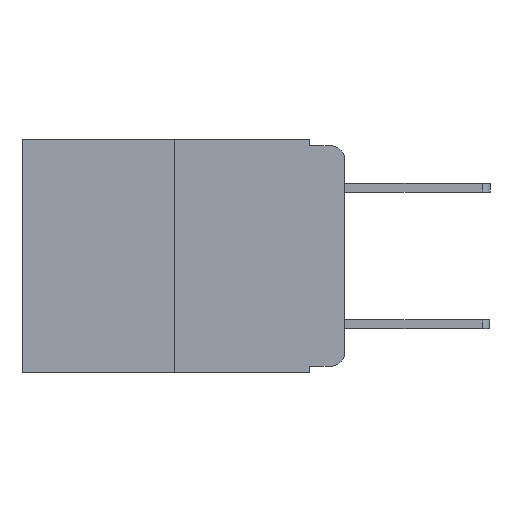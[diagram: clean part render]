
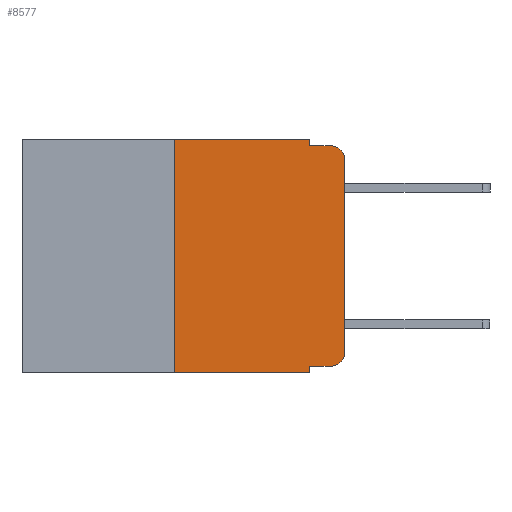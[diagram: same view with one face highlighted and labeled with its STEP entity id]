
A CAD part, left-side view. The second image highlights one B-rep face of the part: STEP entity #8577.
In plain terms, the highlighted planar face has unit normal (-1, 0, 0).
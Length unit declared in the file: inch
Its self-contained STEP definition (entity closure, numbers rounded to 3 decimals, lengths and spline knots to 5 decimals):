
#86 = EDGE_CURVE ( 'NONE', #1387, #10862, #3607, .T. ) ;
#241 = DIRECTION ( 'NONE',  ( 0., 0., -1. ) ) ;
#514 = DIRECTION ( 'NONE',  ( 0., 0., -1. ) ) ;
#557 = DIRECTION ( 'NONE',  ( 0., 0., -1. ) ) ;
#884 = CARTESIAN_POINT ( 'NONE',  ( 0., 0.051, 0. ) ) ;
#912 = VECTOR ( 'NONE', #6676, 39.37008 ) ;
#996 = ORIENTED_EDGE ( 'NONE', *, *, #6839, .F. ) ;
#1213 = LINE ( 'NONE', #5836, #912 ) ;
#1271 = VECTOR ( 'NONE', #1959, 39.37008 ) ;
#1387 = VERTEX_POINT ( 'NONE', #10732 ) ;
#1526 = DIRECTION ( 'NONE',  ( 0., -1., 0. ) ) ;
#1677 = VERTEX_POINT ( 'NONE', #6286 ) ;
#1717 = LINE ( 'NONE', #3192, #10465 ) ;
#1836 = PLANE ( 'NONE',  #3617 ) ;
#1959 = DIRECTION ( 'NONE',  ( 0., 0., 1. ) ) ;
#2155 = DIRECTION ( 'NONE',  ( 0., 0., -1. ) ) ;
#2168 = DIRECTION ( 'NONE',  ( -1., 0., 0. ) ) ;
#2172 = CARTESIAN_POINT ( 'NONE',  ( 0., 0.02, -0.03 ) ) ;
#2195 = CARTESIAN_POINT ( 'NONE',  ( 0., 0.473, 0. ) ) ;
#2405 = CARTESIAN_POINT ( 'NONE',  ( 0., 0.02, -0.333 ) ) ;
#2695 = ORIENTED_EDGE ( 'NONE', *, *, #5338, .T. ) ;
#2699 = VERTEX_POINT ( 'NONE', #2405 ) ;
#2717 = DIRECTION ( 'NONE',  ( 1., 0., 0. ) ) ;
#3094 = ORIENTED_EDGE ( 'NONE', *, *, #5093, .F. ) ;
#3158 = DIRECTION ( 'NONE',  ( -1., 0., 0. ) ) ;
#3192 = CARTESIAN_POINT ( 'NONE',  ( 0., 0.051, 0. ) ) ;
#3607 = LINE ( 'NONE', #884, #5681 ) ;
#3617 = AXIS2_PLACEMENT_3D ( 'NONE', #7880, #2717, #8708 ) ;
#4043 = ORIENTED_EDGE ( 'NONE', *, *, #8713, .F. ) ;
#4108 = CARTESIAN_POINT ( 'NONE',  ( 0., 0.25, 0. ) ) ;
#4157 = EDGE_CURVE ( 'NONE', #6738, #10862, #5843, .T. ) ;
#4356 = EDGE_CURVE ( 'NONE', #8860, #1677, #10583, .T. ) ;
#4397 = CARTESIAN_POINT ( 'NONE',  ( 0., 0., 0. ) ) ;
#4400 = CARTESIAN_POINT ( 'NONE',  ( 0., 0., -0.313 ) ) ;
#4438 = EDGE_CURVE ( 'NONE', #2699, #8860, #5134, .T. ) ;
#4764 = CARTESIAN_POINT ( 'NONE',  ( 0., 0.051, -0.343 ) ) ;
#4814 = VERTEX_POINT ( 'NONE', #4108 ) ;
#4896 = EDGE_LOOP ( 'NONE', ( #10614, #2695, #4043, #8983, #3094, #996, #6770, #7943, #9459, #10344 ) ) ;
#5035 = CARTESIAN_POINT ( 'NONE',  ( 0., 0.051, -0.01 ) ) ;
#5093 = EDGE_CURVE ( 'NONE', #4814, #6397, #6067, .T. ) ;
#5134 = CIRCLE ( 'NONE', #10412, 0.02 ) ;
#5338 = EDGE_CURVE ( 'NONE', #1677, #9386, #5941, .T. ) ;
#5553 = VERTEX_POINT ( 'NONE', #9398 ) ;
#5681 = VECTOR ( 'NONE', #557, 39.37008 ) ;
#5836 = CARTESIAN_POINT ( 'NONE',  ( 0., 0.25, 0. ) ) ;
#5840 = CARTESIAN_POINT ( 'NONE',  ( 0., 0.02, -0.313 ) ) ;
#5843 = LINE ( 'NONE', #6754, #9705 ) ;
#5941 = CIRCLE ( 'NONE', #6530, 0.02 ) ;
#6067 = LINE ( 'NONE', #2195, #10438 ) ;
#6286 = CARTESIAN_POINT ( 'NONE',  ( 0., 0., -0.03 ) ) ;
#6397 = VERTEX_POINT ( 'NONE', #11040 ) ;
#6530 = AXIS2_PLACEMENT_3D ( 'NONE', #2172, #2168, #2155 ) ;
#6539 = CARTESIAN_POINT ( 'NONE',  ( 0., 0.25, -0.343 ) ) ;
#6640 = EDGE_CURVE ( 'NONE', #1387, #2699, #7485, .T. ) ;
#6676 = DIRECTION ( 'NONE',  ( 0., 0., 1. ) ) ;
#6738 = VERTEX_POINT ( 'NONE', #6539 ) ;
#6754 = CARTESIAN_POINT ( 'NONE',  ( 0., 0.473, -0.343 ) ) ;
#6770 = ORIENTED_EDGE ( 'NONE', *, *, #4157, .T. ) ;
#6839 = EDGE_CURVE ( 'NONE', #6738, #4814, #1213, .T. ) ;
#7230 = VECTOR ( 'NONE', #8129, 39.37008 ) ;
#7307 = CARTESIAN_POINT ( 'NONE',  ( 0., 0.051, -0.333 ) ) ;
#7485 = LINE ( 'NONE', #7307, #7230 ) ;
#7732 = CARTESIAN_POINT ( 'NONE',  ( 0., 0.02, -0.01 ) ) ;
#7880 = CARTESIAN_POINT ( 'NONE',  ( 0., 0.473, 0. ) ) ;
#7943 = ORIENTED_EDGE ( 'NONE', *, *, #86, .F. ) ;
#8099 = DIRECTION ( 'NONE',  ( 0., -1., 0. ) ) ;
#8129 = DIRECTION ( 'NONE',  ( 0., -1., 0. ) ) ;
#8577 = ADVANCED_FACE ( 'NONE', ( #9272 ), #1836, .F. ) ;
#8708 = DIRECTION ( 'NONE',  ( 0., 0., -1. ) ) ;
#8713 = EDGE_CURVE ( 'NONE', #5553, #9386, #9887, .T. ) ;
#8860 = VERTEX_POINT ( 'NONE', #4400 ) ;
#8983 = ORIENTED_EDGE ( 'NONE', *, *, #10324, .F. ) ;
#9272 = FACE_OUTER_BOUND ( 'NONE', #4896, .T. ) ;
#9386 = VERTEX_POINT ( 'NONE', #7732 ) ;
#9398 = CARTESIAN_POINT ( 'NONE',  ( 0., 0.051, -0.01 ) ) ;
#9459 = ORIENTED_EDGE ( 'NONE', *, *, #6640, .T. ) ;
#9705 = VECTOR ( 'NONE', #11120, 39.37008 ) ;
#9887 = LINE ( 'NONE', #5035, #10129 ) ;
#10129 = VECTOR ( 'NONE', #1526, 39.37008 ) ;
#10324 = EDGE_CURVE ( 'NONE', #6397, #5553, #1717, .T. ) ;
#10344 = ORIENTED_EDGE ( 'NONE', *, *, #4438, .T. ) ;
#10412 = AXIS2_PLACEMENT_3D ( 'NONE', #5840, #3158, #241 ) ;
#10438 = VECTOR ( 'NONE', #8099, 39.37008 ) ;
#10465 = VECTOR ( 'NONE', #514, 39.37008 ) ;
#10583 = LINE ( 'NONE', #4397, #1271 ) ;
#10614 = ORIENTED_EDGE ( 'NONE', *, *, #4356, .T. ) ;
#10732 = CARTESIAN_POINT ( 'NONE',  ( 0., 0.051, -0.333 ) ) ;
#10862 = VERTEX_POINT ( 'NONE', #4764 ) ;
#11040 = CARTESIAN_POINT ( 'NONE',  ( 0., 0.051, 0. ) ) ;
#11120 = DIRECTION ( 'NONE',  ( 0., -1., 0. ) ) ;
